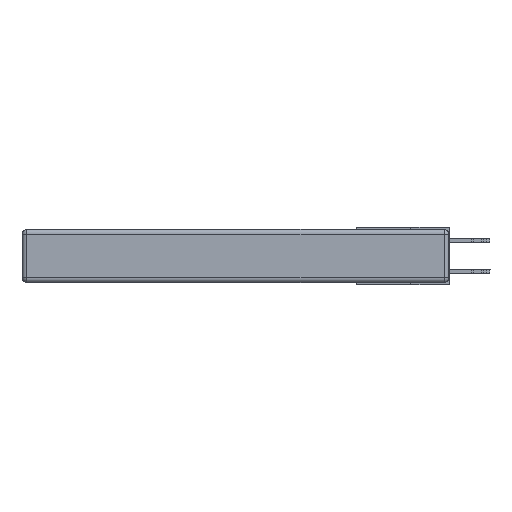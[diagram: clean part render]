
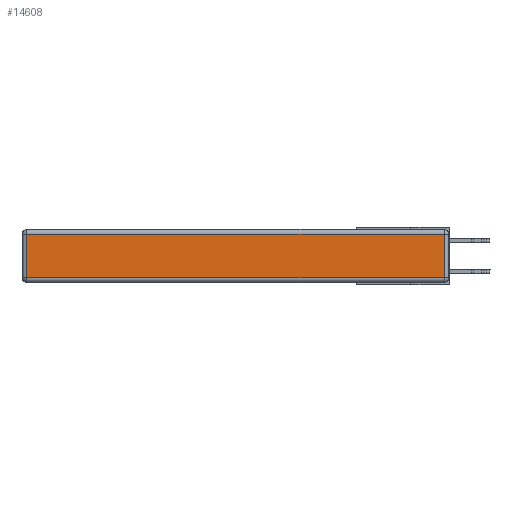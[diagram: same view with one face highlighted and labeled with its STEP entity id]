
A CAD part, left-side view. The second image highlights one B-rep face of the part: STEP entity #14608.
In plain terms, the highlighted planar face has unit normal (-1, 0, 0).
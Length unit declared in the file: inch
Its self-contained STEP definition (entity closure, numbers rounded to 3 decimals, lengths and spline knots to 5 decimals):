
#316 = AXIS2_PLACEMENT_3D ( 'NONE', #14553, #9608, #21895 ) ;
#955 = EDGE_CURVE ( 'NONE', #16766, #1675, #17572, .T. ) ;
#1675 = VERTEX_POINT ( 'NONE', #29095 ) ;
#2119 = VERTEX_POINT ( 'NONE', #8563 ) ;
#5335 = LINE ( 'NONE', #20437, #25111 ) ;
#6735 = ORIENTED_EDGE ( 'NONE', *, *, #17540, .T. ) ;
#7674 = ORIENTED_EDGE ( 'NONE', *, *, #955, .T. ) ;
#7815 = LINE ( 'NONE', #11094, #15307 ) ;
#7982 = CARTESIAN_POINT ( 'NONE',  ( 0., 0.03, -0.313 ) ) ;
#8563 = CARTESIAN_POINT ( 'NONE',  ( 0., 2.72, -0.313 ) ) ;
#9608 = DIRECTION ( 'NONE',  ( -1., 0., 0. ) ) ;
#10442 = DIRECTION ( 'NONE',  ( 0., 1., 0. ) ) ;
#10662 = CARTESIAN_POINT ( 'NONE',  ( 0., 2.72, -0.343 ) ) ;
#11094 = CARTESIAN_POINT ( 'NONE',  ( 0., 0., -0.313 ) ) ;
#12986 = DIRECTION ( 'NONE',  ( 0., 0., -1. ) ) ;
#13760 = DIRECTION ( 'NONE',  ( 0., -1., 0. ) ) ;
#14553 = CARTESIAN_POINT ( 'NONE',  ( 0., 0., -0.343 ) ) ;
#14608 = ADVANCED_FACE ( 'NONE', ( #15930 ), #31555, .T. ) ;
#15307 = VECTOR ( 'NONE', #13760, 39.37008 ) ;
#15930 = FACE_OUTER_BOUND ( 'NONE', #30983, .T. ) ;
#15962 = VECTOR ( 'NONE', #10442, 39.37008 ) ;
#16331 = VECTOR ( 'NONE', #12986, 39.37008 ) ;
#16766 = VERTEX_POINT ( 'NONE', #20512 ) ;
#17540 = EDGE_CURVE ( 'NONE', #1675, #2119, #31311, .T. ) ;
#17572 = LINE ( 'NONE', #22213, #15962 ) ;
#19050 = EDGE_CURVE ( 'NONE', #2119, #22322, #7815, .T. ) ;
#20437 = CARTESIAN_POINT ( 'NONE',  ( 0., 0.03, -0.343 ) ) ;
#20512 = CARTESIAN_POINT ( 'NONE',  ( 0., 0.03, -0.03 ) ) ;
#21725 = ORIENTED_EDGE ( 'NONE', *, *, #19050, .T. ) ;
#21895 = DIRECTION ( 'NONE',  ( 0., 0., 1. ) ) ;
#22213 = CARTESIAN_POINT ( 'NONE',  ( 0., 2.75, -0.03 ) ) ;
#22322 = VERTEX_POINT ( 'NONE', #7982 ) ;
#24295 = ORIENTED_EDGE ( 'NONE', *, *, #25752, .T. ) ;
#25111 = VECTOR ( 'NONE', #30475, 39.37008 ) ;
#25752 = EDGE_CURVE ( 'NONE', #22322, #16766, #5335, .T. ) ;
#29095 = CARTESIAN_POINT ( 'NONE',  ( 0., 2.72, -0.03 ) ) ;
#30475 = DIRECTION ( 'NONE',  ( 0., 0., 1. ) ) ;
#30983 = EDGE_LOOP ( 'NONE', ( #21725, #24295, #7674, #6735 ) ) ;
#31311 = LINE ( 'NONE', #10662, #16331 ) ;
#31555 = PLANE ( 'NONE',  #316 ) ;
